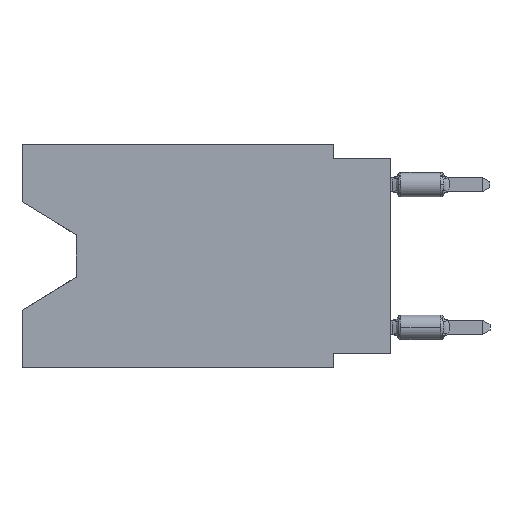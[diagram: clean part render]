
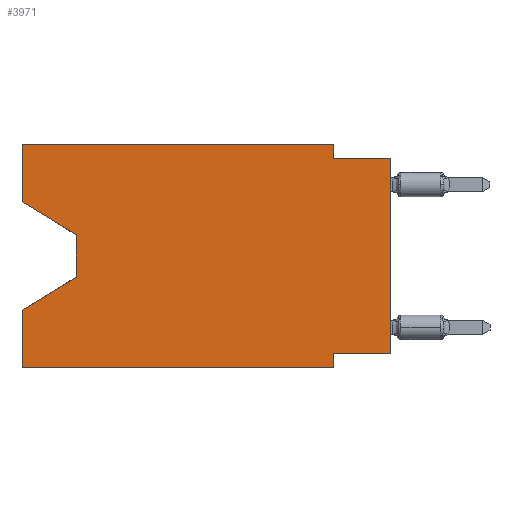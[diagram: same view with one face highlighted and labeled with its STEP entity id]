
A CAD part, left-side view. The second image highlights one B-rep face of the part: STEP entity #3971.
In plain terms, the highlighted planar face has unit normal (-1, 0, 0).
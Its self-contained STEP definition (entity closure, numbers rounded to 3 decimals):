
#33 = DIRECTION ( 'NONE',  ( 0., -1., 0. ) ) ;
#77 = LINE ( 'NONE', #6725, #10325 ) ;
#153 = DIRECTION ( 'NONE',  ( 0., 0.855, -0.519 ) ) ;
#350 = VERTEX_POINT ( 'NONE', #5524 ) ;
#495 = FACE_OUTER_BOUND ( 'NONE', #4326, .T. ) ;
#555 = VECTOR ( 'NONE', #13391, 1000. ) ;
#795 = DIRECTION ( 'NONE',  ( 0., 1., 0. ) ) ;
#933 = EDGE_CURVE ( 'NONE', #9805, #2918, #7227, .T. ) ;
#950 = CARTESIAN_POINT ( 'NONE',  ( 0., 13.97, -4.013 ) ) ;
#1010 = VERTEX_POINT ( 'NONE', #7370 ) ;
#1317 = VERTEX_POINT ( 'NONE', #1811 ) ;
#1660 = CARTESIAN_POINT ( 'NONE',  ( 0., 16.383, 0. ) ) ;
#1706 = LINE ( 'NONE', #3903, #11004 ) ;
#1757 = CARTESIAN_POINT ( 'NONE',  ( 0., 0., -9.271 ) ) ;
#1811 = CARTESIAN_POINT ( 'NONE',  ( 0., 16.383, -2.546 ) ) ;
#1870 = CARTESIAN_POINT ( 'NONE',  ( 0., 2.54, 0. ) ) ;
#1895 = EDGE_CURVE ( 'NONE', #2918, #3733, #10943, .T. ) ;
#2371 = ORIENTED_EDGE ( 'NONE', *, *, #3240, .T. ) ;
#2585 = DIRECTION ( 'NONE',  ( 0., 0., 1. ) ) ;
#2859 = ORIENTED_EDGE ( 'NONE', *, *, #14167, .F. ) ;
#2918 = VERTEX_POINT ( 'NONE', #6244 ) ;
#3007 = LINE ( 'NONE', #14195, #8098 ) ;
#3092 = CARTESIAN_POINT ( 'NONE',  ( 0., 2.54, 0. ) ) ;
#3240 = EDGE_CURVE ( 'NONE', #3431, #3733, #7038, .T. ) ;
#3426 = EDGE_CURVE ( 'NONE', #350, #7695, #5788, .T. ) ;
#3431 = VERTEX_POINT ( 'NONE', #8100 ) ;
#3650 = VECTOR ( 'NONE', #153, 1000. ) ;
#3733 = VERTEX_POINT ( 'NONE', #13374 ) ;
#3879 = VERTEX_POINT ( 'NONE', #13724 ) ;
#3891 = DIRECTION ( 'NONE',  ( 0., -1., 0. ) ) ;
#3903 = CARTESIAN_POINT ( 'NONE',  ( 0., 0., 0. ) ) ;
#3971 = ADVANCED_FACE ( 'NONE', ( #495 ), #9373, .F. ) ;
#4003 = CARTESIAN_POINT ( 'NONE',  ( 0., 16.383, -7.36 ) ) ;
#4038 = DIRECTION ( 'NONE',  ( 0., 0., 1. ) ) ;
#4316 = LINE ( 'NONE', #950, #555 ) ;
#4326 = EDGE_LOOP ( 'NONE', ( #7344, #7042, #7750, #2859, #2371, #9968, #4554, #11940, #13659, #8261, #6312, #8340 ) ) ;
#4554 = ORIENTED_EDGE ( 'NONE', *, *, #933, .F. ) ;
#4585 = VECTOR ( 'NONE', #3891, 1000. ) ;
#4642 = VECTOR ( 'NONE', #795, 1000. ) ;
#4702 = EDGE_CURVE ( 'NONE', #1010, #10270, #4766, .T. ) ;
#4766 = LINE ( 'NONE', #7240, #4585 ) ;
#5200 = VECTOR ( 'NONE', #8877, 1000. ) ;
#5415 = CARTESIAN_POINT ( 'NONE',  ( 0., 16.383, 0. ) ) ;
#5524 = CARTESIAN_POINT ( 'NONE',  ( 0., 13.97, -5.893 ) ) ;
#5610 = LINE ( 'NONE', #6705, #5200 ) ;
#5657 = EDGE_CURVE ( 'NONE', #10270, #7582, #9637, .T. ) ;
#5788 = LINE ( 'NONE', #13538, #3650 ) ;
#5983 = VECTOR ( 'NONE', #8561, 1000. ) ;
#6110 = DIRECTION ( 'NONE',  ( 1., 0., 0. ) ) ;
#6236 = VECTOR ( 'NONE', #4038, 1000. ) ;
#6244 = CARTESIAN_POINT ( 'NONE',  ( 0., 2.54, -9.271 ) ) ;
#6312 = ORIENTED_EDGE ( 'NONE', *, *, #4702, .F. ) ;
#6509 = LINE ( 'NONE', #5415, #6236 ) ;
#6705 = CARTESIAN_POINT ( 'NONE',  ( 0., 0., -0.635 ) ) ;
#6725 = CARTESIAN_POINT ( 'NONE',  ( 0., 16.383, 0. ) ) ;
#6899 = CARTESIAN_POINT ( 'NONE',  ( 0., 16.383, -9.906 ) ) ;
#7038 = LINE ( 'NONE', #6899, #8284 ) ;
#7042 = ORIENTED_EDGE ( 'NONE', *, *, #14184, .T. ) ;
#7227 = LINE ( 'NONE', #1757, #4642 ) ;
#7240 = CARTESIAN_POINT ( 'NONE',  ( 0., 16.383, 0. ) ) ;
#7344 = ORIENTED_EDGE ( 'NONE', *, *, #8037, .T. ) ;
#7370 = CARTESIAN_POINT ( 'NONE',  ( 0., 16.383, 0. ) ) ;
#7582 = VERTEX_POINT ( 'NONE', #8437 ) ;
#7613 = DIRECTION ( 'NONE',  ( 0., 0., -1. ) ) ;
#7695 = VERTEX_POINT ( 'NONE', #4003 ) ;
#7733 = DIRECTION ( 'NONE',  ( 0., 0., 1. ) ) ;
#7750 = ORIENTED_EDGE ( 'NONE', *, *, #3426, .T. ) ;
#8037 = EDGE_CURVE ( 'NONE', #1317, #3879, #3007, .T. ) ;
#8042 = AXIS2_PLACEMENT_3D ( 'NONE', #1660, #6110, #8361 ) ;
#8065 = EDGE_CURVE ( 'NONE', #1317, #1010, #6509, .T. ) ;
#8098 = VECTOR ( 'NONE', #12025, 1000. ) ;
#8100 = CARTESIAN_POINT ( 'NONE',  ( 0., 16.383, -9.906 ) ) ;
#8231 = CARTESIAN_POINT ( 'NONE',  ( 0., 0., -9.271 ) ) ;
#8261 = ORIENTED_EDGE ( 'NONE', *, *, #5657, .F. ) ;
#8284 = VECTOR ( 'NONE', #33, 1000. ) ;
#8340 = ORIENTED_EDGE ( 'NONE', *, *, #8065, .F. ) ;
#8361 = DIRECTION ( 'NONE',  ( 0., 0., -1. ) ) ;
#8374 = CARTESIAN_POINT ( 'NONE',  ( 0., 0., -0.635 ) ) ;
#8437 = CARTESIAN_POINT ( 'NONE',  ( 0., 2.54, -0.635 ) ) ;
#8561 = DIRECTION ( 'NONE',  ( 0., 0., -1. ) ) ;
#8877 = DIRECTION ( 'NONE',  ( 0., -1., 0. ) ) ;
#9201 = VECTOR ( 'NONE', #7613, 1000. ) ;
#9373 = PLANE ( 'NONE',  #8042 ) ;
#9637 = LINE ( 'NONE', #3092, #9201 ) ;
#9783 = CARTESIAN_POINT ( 'NONE',  ( 0., 2.54, -9.906 ) ) ;
#9805 = VERTEX_POINT ( 'NONE', #8231 ) ;
#9968 = ORIENTED_EDGE ( 'NONE', *, *, #1895, .F. ) ;
#10270 = VERTEX_POINT ( 'NONE', #1870 ) ;
#10325 = VECTOR ( 'NONE', #7733, 1000. ) ;
#10943 = LINE ( 'NONE', #9783, #5983 ) ;
#11004 = VECTOR ( 'NONE', #2585, 1000. ) ;
#11940 = ORIENTED_EDGE ( 'NONE', *, *, #13543, .T. ) ;
#12025 = DIRECTION ( 'NONE',  ( 0., -0.855, -0.519 ) ) ;
#12685 = VERTEX_POINT ( 'NONE', #8374 ) ;
#12953 = EDGE_CURVE ( 'NONE', #7582, #12685, #5610, .T. ) ;
#13374 = CARTESIAN_POINT ( 'NONE',  ( 0., 2.54, -9.906 ) ) ;
#13391 = DIRECTION ( 'NONE',  ( 0., 0., -1. ) ) ;
#13538 = CARTESIAN_POINT ( 'NONE',  ( 0., 13.97, -5.893 ) ) ;
#13543 = EDGE_CURVE ( 'NONE', #9805, #12685, #1706, .T. ) ;
#13659 = ORIENTED_EDGE ( 'NONE', *, *, #12953, .F. ) ;
#13724 = CARTESIAN_POINT ( 'NONE',  ( 0., 13.97, -4.013 ) ) ;
#14167 = EDGE_CURVE ( 'NONE', #3431, #7695, #77, .T. ) ;
#14184 = EDGE_CURVE ( 'NONE', #3879, #350, #4316, .T. ) ;
#14195 = CARTESIAN_POINT ( 'NONE',  ( 0., 16.383, -2.546 ) ) ;
